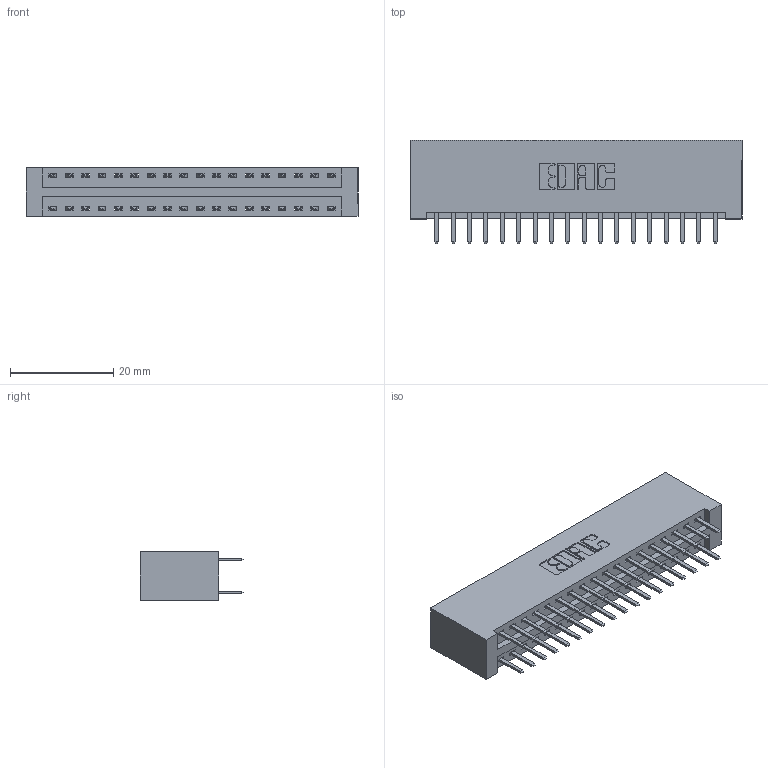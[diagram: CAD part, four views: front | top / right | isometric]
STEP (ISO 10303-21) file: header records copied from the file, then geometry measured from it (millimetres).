
FILE_DESCRIPTION (( 'STEP AP203' ), '1' );
FILE_NAME ('396-036-520-201.STEP', '2018-09-06T03:11:33', ( '' ), ( '' ), 'SwSTEP 2.0', 'SolidWorks 2016', '' );
FILE_SCHEMA (( 'CONFIG_CONTROL_DESIGN' ));
Length unit declared in the file: inch
Products named in the file (3): 345-292-001_345-293-120; 396-036-520-201; 346 Part_No Mounting Lugs
Assembly tree (37 placements, depth 2):
  396-036-520-201
    346 Part_No Mounting Lugs
    345-292-001_345-293-120  x36
Bounding box: 64.39 x 20.02 x 9.4 mm (x, y, z)
Volume: 6649.8 mm3; surface area: 8889.5 mm2
Topology: 37 solids, 37 shells, 2130 faces, 6173 edges, 4018 vertices
Faces by surface type: plane 1404, cylinder 726
Entity records: 14815 total; most frequent: CARTESIAN_POINT 2484, ORIENTED_EDGE 2406, DIRECTION 2223, EDGE_CURVE 1203, LINE 1003, VECTOR 1003, VERTEX_POINT 798, AXIS2_PLACEMENT_3D 610
